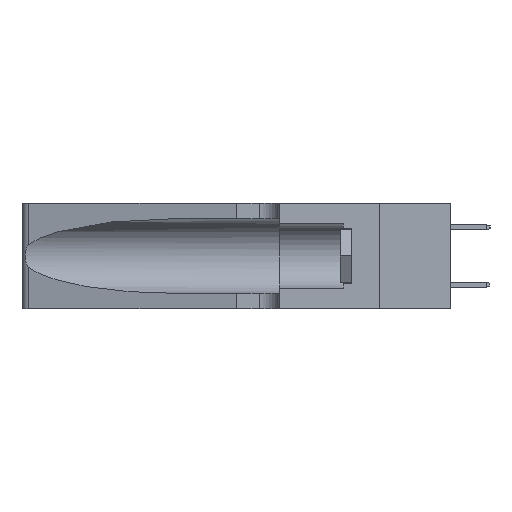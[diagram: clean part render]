
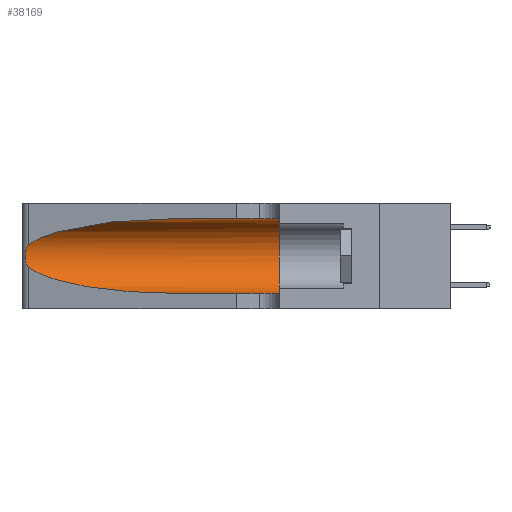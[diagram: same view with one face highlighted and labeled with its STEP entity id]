
A CAD part, left-side view. The second image highlights one B-rep face of the part: STEP entity #38169.
In plain terms, the highlighted cylindrical face has radius 3.308 mm (diameter 6.617 mm), a partial arc.
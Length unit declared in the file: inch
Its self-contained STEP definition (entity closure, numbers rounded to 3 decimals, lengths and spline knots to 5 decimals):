
#446 = CARTESIAN_POINT ( 'NONE',  ( 0.1305, 0.35, 0.05475 ) ) ;
#581 = CARTESIAN_POINT ( 'NONE',  ( 0.25555, 1.22994, 0.2215 ) ) ;
#2961 = EDGE_CURVE ( 'NONE', #36323, #34891, #6350, .T. ) ;
#3987 = VECTOR ( 'NONE', #24029, 39.37008 ) ;
#4489 = CARTESIAN_POINT ( 'NONE',  ( 0.26075, 1.23896, 0.19203 ) ) ;
#4656 = FACE_OUTER_BOUND ( 'NONE', #36856, .T. ) ;
#5032 = EDGE_CURVE ( 'NONE', #35915, #36323, #43686, .T. ) ;
#5637 = DIRECTION ( 'NONE',  ( 0., -1., 0. ) ) ;
#6228 = ORIENTED_EDGE ( 'NONE', *, *, #35230, .F. ) ;
#6350 =( BOUNDED_CURVE ( )  B_SPLINE_CURVE ( 3, ( #21872, #14832, #19437, #34336 ),
 .UNSPECIFIED., .F., .T. ) 
 B_SPLINE_CURVE_WITH_KNOTS ( ( 4, 4 ),
 ( 3.44316, 4.71239 ),
 .UNSPECIFIED. ) 
 CURVE ( )  GEOMETRIC_REPRESENTATION_ITEM ( )  RATIONAL_B_SPLINE_CURVE ( ( 1., 0.87, 0.87, 1. ) ) 
 REPRESENTATION_ITEM ( '' )  );
#6936 = ORIENTED_EDGE ( 'NONE', *, *, #29297, .F. ) ;
#8006 = VECTOR ( 'NONE', #5637, 39.37008 ) ;
#8385 = CARTESIAN_POINT ( 'NONE',  ( 0.25555, 1.22993, 0.14849 ) ) ;
#8861 = CARTESIAN_POINT ( 'NONE',  ( 0.25639, 1.23184, 0.21858 ) ) ;
#9170 = CARTESIAN_POINT ( 'NONE',  ( 0.1305, 1.61858, 0.05475 ) ) ;
#10097 = CARTESIAN_POINT ( 'NONE',  ( 0.25487, 1.22718, 0.22369 ) ) ;
#11002 = CARTESIAN_POINT ( 'NONE',  ( 0.25487, 1.22718, 0.22369 ) ) ;
#11796 = CARTESIAN_POINT ( 'NONE',  ( 0.25639, 1.23186, 0.15144 ) ) ;
#12272 = CARTESIAN_POINT ( 'NONE',  ( 0.25487, 1.22718, 0.22369 ) ) ;
#12349 = DIRECTION ( 'NONE',  ( 0., 1., 0. ) ) ;
#14664 = CARTESIAN_POINT ( 'NONE',  ( 0.18966, 0.96281, 0.31525 ) ) ;
#14832 = CARTESIAN_POINT ( 'NONE',  ( 0.2373, 1.15595, 0.08982 ) ) ;
#16074 = VERTEX_POINT ( 'NONE', #37558 ) ;
#16797 = EDGE_CURVE ( 'NONE', #34891, #22795, #17437, .T. ) ;
#17437 = LINE ( 'NONE', #9170, #3987 ) ;
#18111 = CARTESIAN_POINT ( 'NONE',  ( 0.1305, 0.35, 0.31525 ) ) ;
#19437 = CARTESIAN_POINT ( 'NONE',  ( 0.18966, 0.96281, 0.05475 ) ) ;
#20346 = ORIENTED_EDGE ( 'NONE', *, *, #36666, .T. ) ;
#20446 = CIRCLE ( 'NONE', #25939, 0.13025 ) ;
#20943 = CYLINDRICAL_SURFACE ( 'NONE', #40864, 0.13025 ) ;
#21420 = DIRECTION ( 'NONE',  ( 0., -1., 0. ) ) ;
#21571 =( BOUNDED_CURVE ( )  B_SPLINE_CURVE ( 3, ( #36852, #14664, #29540, #11002 ),
 .UNSPECIFIED., .F., .F. ) 
 B_SPLINE_CURVE_WITH_KNOTS ( ( 4, 4 ),
 ( 1.5708, 2.84003 ),
 .UNSPECIFIED. ) 
 CURVE ( )  GEOMETRIC_REPRESENTATION_ITEM ( )  RATIONAL_B_SPLINE_CURVE ( ( 1., 0.87, 0.87, 1. ) ) 
 REPRESENTATION_ITEM ( '' )  );
#21872 = CARTESIAN_POINT ( 'NONE',  ( 0.25487, 1.22718, 0.14631 ) ) ;
#22751 = CARTESIAN_POINT ( 'NONE',  ( 0.25856, 1.23593, 0.16098 ) ) ;
#22795 = VERTEX_POINT ( 'NONE', #446 ) ;
#23235 = CARTESIAN_POINT ( 'NONE',  ( 0.25487, 1.22718, 0.14631 ) ) ;
#23464 = CARTESIAN_POINT ( 'NONE',  ( 0.25854, 1.2359, 0.20912 ) ) ;
#23715 = CARTESIAN_POINT ( 'NONE',  ( 0.26018, 1.23835, 0.19895 ) ) ;
#24029 = DIRECTION ( 'NONE',  ( 0., -1., 0. ) ) ;
#24508 = CARTESIAN_POINT ( 'NONE',  ( 0.1305, 0.35, 0.185 ) ) ;
#24811 = ORIENTED_EDGE ( 'NONE', *, *, #5032, .T. ) ;
#24860 = CARTESIAN_POINT ( 'NONE',  ( 0.1305, 1.61858, 0.185 ) ) ;
#24894 = LINE ( 'NONE', #28564, #8006 ) ;
#25939 = AXIS2_PLACEMENT_3D ( 'NONE', #24508, #12349, #42842 ) ;
#27151 = CARTESIAN_POINT ( 'NONE',  ( 0.25789, 1.23486, 0.15765 ) ) ;
#27378 = CARTESIAN_POINT ( 'NONE',  ( 0.26017, 1.23833, 0.17102 ) ) ;
#28564 = CARTESIAN_POINT ( 'NONE',  ( 0.1305, 1.61858, 0.31525 ) ) ;
#29297 = EDGE_CURVE ( 'NONE', #46279, #22795, #20446, .T. ) ;
#29540 = CARTESIAN_POINT ( 'NONE',  ( 0.2373, 1.15595, 0.28018 ) ) ;
#33979 = CARTESIAN_POINT ( 'NONE',  ( 0.1305, 0.72297, 0.05475 ) ) ;
#34336 = CARTESIAN_POINT ( 'NONE',  ( 0.1305, 0.72297, 0.05475 ) ) ;
#34891 = VERTEX_POINT ( 'NONE', #33979 ) ;
#35230 = EDGE_CURVE ( 'NONE', #16074, #46279, #24894, .T. ) ;
#35915 = VERTEX_POINT ( 'NONE', #10097 ) ;
#36323 = VERTEX_POINT ( 'NONE', #38341 ) ;
#36331 = DIRECTION ( 'NONE',  ( 0., 0., -1. ) ) ;
#36666 = EDGE_CURVE ( 'NONE', #16074, #35915, #21571, .T. ) ;
#36852 = CARTESIAN_POINT ( 'NONE',  ( 0.1305, 0.72297, 0.31525 ) ) ;
#36856 = EDGE_LOOP ( 'NONE', ( #20346, #24811, #39261, #37438, #6936, #6228 ) ) ;
#37438 = ORIENTED_EDGE ( 'NONE', *, *, #16797, .T. ) ;
#37558 = CARTESIAN_POINT ( 'NONE',  ( 0.1305, 0.72297, 0.31525 ) ) ;
#38169 = ADVANCED_FACE ( 'NONE', ( #4656 ), #20943, .F. ) ;
#38341 = CARTESIAN_POINT ( 'NONE',  ( 0.25487, 1.22718, 0.14631 ) ) ;
#39261 = ORIENTED_EDGE ( 'NONE', *, *, #2961, .T. ) ;
#40864 = AXIS2_PLACEMENT_3D ( 'NONE', #24860, #21420, #36331 ) ;
#41814 = CARTESIAN_POINT ( 'NONE',  ( 0.26075, 1.23896, 0.178 ) ) ;
#42842 = DIRECTION ( 'NONE',  ( 0., 0., 1. ) ) ;
#43686 = B_SPLINE_CURVE_WITH_KNOTS ( 'NONE', 3,
 ( #12272, #581, #8861, #45240, #23464, #23715, #4489, #41814, #27378, #22751, #27151, #11796, #8385, #23235 ),
 .UNSPECIFIED., .F., .F.,
 ( 4, 2, 2, 2, 2, 2, 4 ),
 ( 0., 0.00027, 0.00053, 0.00107, 0.0016, 0.00187, 0.00214 ),
 .UNSPECIFIED. ) ;
#45240 = CARTESIAN_POINT ( 'NONE',  ( 0.25787, 1.23484, 0.2124 ) ) ;
#46279 = VERTEX_POINT ( 'NONE', #18111 ) ;
